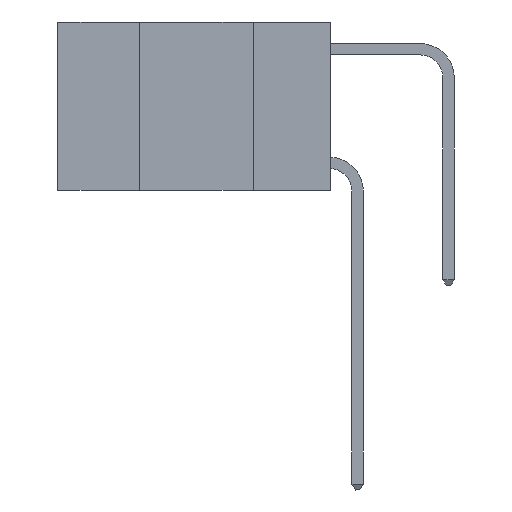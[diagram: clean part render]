
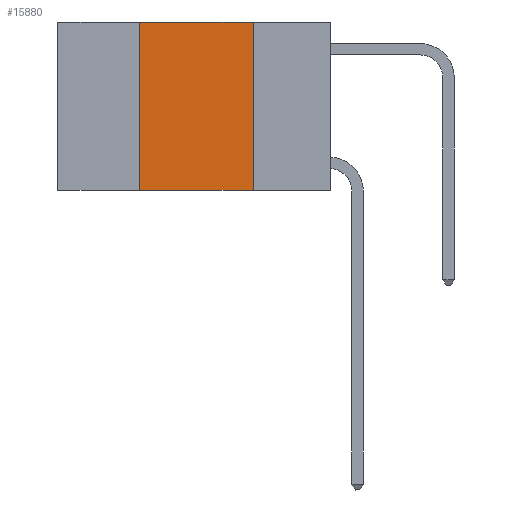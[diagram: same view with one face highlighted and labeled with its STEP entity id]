
A CAD part, left-side view. The second image highlights one B-rep face of the part: STEP entity #15880.
In plain terms, the highlighted planar face has unit normal (-1, 0, 0).
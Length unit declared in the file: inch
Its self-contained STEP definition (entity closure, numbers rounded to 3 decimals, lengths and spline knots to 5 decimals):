
#1085 = ORIENTED_EDGE ( 'NONE', *, *, #4688, .F. ) ;
#1205 = VERTEX_POINT ( 'NONE', #10412 ) ;
#1685 = VERTEX_POINT ( 'NONE', #4627 ) ;
#1869 = VECTOR ( 'NONE', #5122, 39.37008 ) ;
#3031 = VERTEX_POINT ( 'NONE', #4526 ) ;
#3250 = VECTOR ( 'NONE', #7763, 39.37008 ) ;
#3977 = EDGE_LOOP ( 'NONE', ( #1085, #11636, #6371, #15678 ) ) ;
#3992 = VECTOR ( 'NONE', #16633, 39.37008 ) ;
#4463 = PLANE ( 'NONE',  #16177 ) ;
#4526 = CARTESIAN_POINT ( 'NONE',  ( 0., 0.17, -0.37 ) ) ;
#4627 = CARTESIAN_POINT ( 'NONE',  ( 0., 0.42, -0.37 ) ) ;
#4688 = EDGE_CURVE ( 'NONE', #1205, #3031, #7092, .T. ) ;
#5122 = DIRECTION ( 'NONE',  ( 0., -1., 0. ) ) ;
#6371 = ORIENTED_EDGE ( 'NONE', *, *, #15514, .F. ) ;
#7092 = LINE ( 'NONE', #15856, #16506 ) ;
#7433 = DIRECTION ( 'NONE',  ( 0., 0., -1. ) ) ;
#7714 = CARTESIAN_POINT ( 'NONE',  ( 0., 0.42, 0. ) ) ;
#7763 = DIRECTION ( 'NONE',  ( 0., 0., 1. ) ) ;
#9203 = LINE ( 'NONE', #15177, #3992 ) ;
#9374 = EDGE_CURVE ( 'NONE', #1685, #3031, #9203, .T. ) ;
#9945 = EDGE_CURVE ( 'NONE', #14445, #1205, #16776, .T. ) ;
#10322 = CARTESIAN_POINT ( 'NONE',  ( 0., 0.6, 0. ) ) ;
#10412 = CARTESIAN_POINT ( 'NONE',  ( 0., 0.17, 0. ) ) ;
#11636 = ORIENTED_EDGE ( 'NONE', *, *, #9945, .F. ) ;
#11717 = DIRECTION ( 'NONE',  ( 0., 0., -1. ) ) ;
#12476 = CARTESIAN_POINT ( 'NONE',  ( 0., 0.42, 0. ) ) ;
#13547 = LINE ( 'NONE', #12476, #3250 ) ;
#13595 = CARTESIAN_POINT ( 'NONE',  ( 0., 0.6, 0. ) ) ;
#14445 = VERTEX_POINT ( 'NONE', #7714 ) ;
#15177 = CARTESIAN_POINT ( 'NONE',  ( 0., 0.6, -0.37 ) ) ;
#15514 = EDGE_CURVE ( 'NONE', #1685, #14445, #13547, .T. ) ;
#15678 = ORIENTED_EDGE ( 'NONE', *, *, #9374, .T. ) ;
#15856 = CARTESIAN_POINT ( 'NONE',  ( 0., 0.17, 0. ) ) ;
#15880 = ADVANCED_FACE ( 'NONE', ( #17647 ), #4463, .F. ) ;
#16177 = AXIS2_PLACEMENT_3D ( 'NONE', #10322, #16205, #7433 ) ;
#16205 = DIRECTION ( 'NONE',  ( 1., 0., 0. ) ) ;
#16506 = VECTOR ( 'NONE', #11717, 39.37008 ) ;
#16633 = DIRECTION ( 'NONE',  ( 0., -1., 0. ) ) ;
#16776 = LINE ( 'NONE', #13595, #1869 ) ;
#17647 = FACE_OUTER_BOUND ( 'NONE', #3977, .T. ) ;
